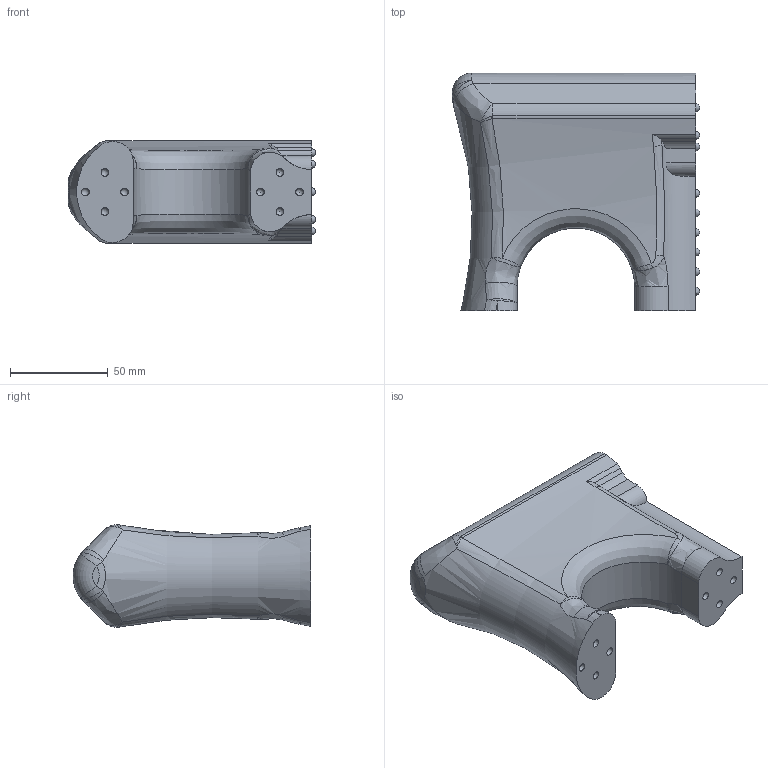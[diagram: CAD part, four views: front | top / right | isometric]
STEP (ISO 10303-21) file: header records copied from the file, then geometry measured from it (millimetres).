
FILE_DESCRIPTION (( 'STEP AP214' ), '1' );
FILE_NAME ('Stock_Rear_V2.step', '2016-01-25T18:17:31', ( 'WarFairy' ), ( '' ), 'SwSTEP 2.0', 'SolidWorks 2015', '' );
FILE_SCHEMA (( 'AUTOMOTIVE_DESIGN' ));
Length unit declared in the file: millimetre
Products named in the file (1): Stock_Rear_V2
Bounding box: 126.29 x 121.45 x 52.5 mm (x, y, z)
Volume: 438681.5 mm3; surface area: 48053.5 mm2
Topology: 1 solids, 1 shells, 98 faces, 279 edges, 165 vertices
Faces by surface type: bspline 31, sphere 27, cylinder 23, plane 13, torus 4
Full cylindrical faces by diameter (mm): 25.654 x1
Entity records: 5216 total; most frequent: CARTESIAN_POINT 3299, ORIENTED_EDGE 410, DIRECTION 339, EDGE_CURVE 205, AXIS2_PLACEMENT_3D 149, VERTEX_POINT 130, EDGE_LOOP 119, FACE_OUTER_BOUND 99
